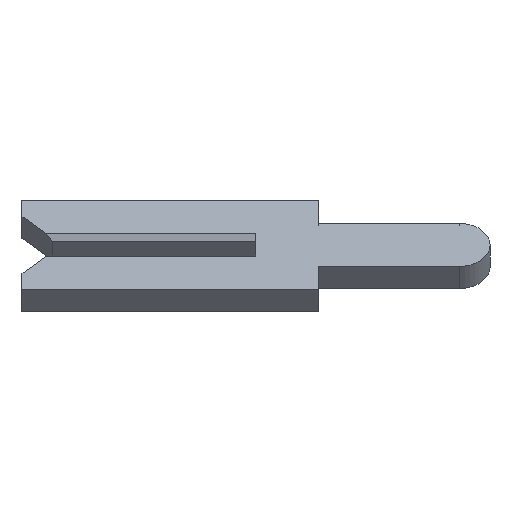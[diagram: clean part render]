
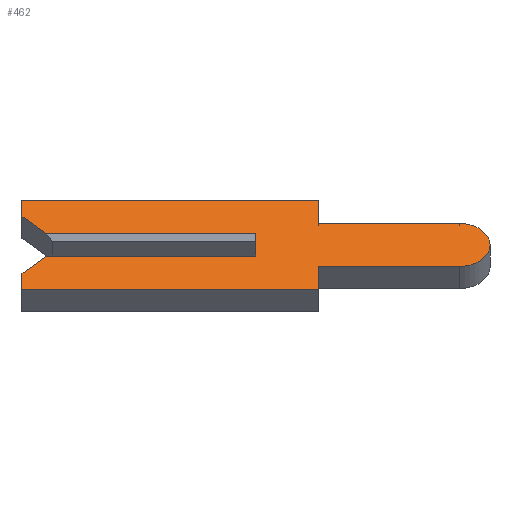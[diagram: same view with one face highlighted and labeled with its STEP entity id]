
A CAD part, left-side view. The second image highlights one B-rep face of the part: STEP entity #462.
In plain terms, the highlighted face is planar.
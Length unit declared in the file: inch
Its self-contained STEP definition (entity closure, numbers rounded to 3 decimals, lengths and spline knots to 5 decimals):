
#1 = VECTOR ( 'NONE', #434, 39.37008 ) ;
#3 = VERTEX_POINT ( 'NONE', #767 ) ;
#26 = ORIENTED_EDGE ( 'NONE', *, *, #602, .F. ) ;
#40 = CIRCLE ( 'NONE', #353, 0.0195 ) ;
#43 = VERTEX_POINT ( 'NONE', #74 ) ;
#44 = ORIENTED_EDGE ( 'NONE', *, *, #184, .F. ) ;
#53 = LINE ( 'NONE', #195, #673 ) ;
#74 = CARTESIAN_POINT ( 'NONE',  ( -0.01, 0.15, 0.04 ) ) ;
#82 = VERTEX_POINT ( 'NONE', #422 ) ;
#83 = CARTESIAN_POINT ( 'NONE',  ( -0.01, 0., 0.0065 ) ) ;
#100 = VECTOR ( 'NONE', #306, 39.37008 ) ;
#101 = ORIENTED_EDGE ( 'NONE', *, *, #229, .F. ) ;
#118 = AXIS2_PLACEMENT_3D ( 'NONE', #884, #601, #881 ) ;
#122 = VECTOR ( 'NONE', #298, 39.37008 ) ;
#135 = VERTEX_POINT ( 'NONE', #213 ) ;
#138 = CARTESIAN_POINT ( 'NONE',  ( -0.01, -0.1305, -0.0195 ) ) ;
#170 = VERTEX_POINT ( 'NONE', #138 ) ;
#176 = VECTOR ( 'NONE', #814, 39.37008 ) ;
#178 = CARTESIAN_POINT ( 'NONE',  ( -0.01, 0., 0.01 ) ) ;
#182 = VERTEX_POINT ( 'NONE', #630 ) ;
#184 = EDGE_CURVE ( 'NONE', #135, #82, #272, .T. ) ;
#185 = LINE ( 'NONE', #519, #402 ) ;
#188 = DIRECTION ( 'NONE',  ( 0., 0., -1. ) ) ;
#191 = ORIENTED_EDGE ( 'NONE', *, *, #483, .F. ) ;
#195 = CARTESIAN_POINT ( 'NONE',  ( -0.01, 0.15, -0.026 ) ) ;
#213 = CARTESIAN_POINT ( 'NONE',  ( -0.01, -0.04, 0.0195 ) ) ;
#216 = ORIENTED_EDGE ( 'NONE', *, *, #458, .F. ) ;
#226 = VERTEX_POINT ( 'NONE', #854 ) ;
#229 = EDGE_CURVE ( 'NONE', #720, #135, #419, .T. ) ;
#232 = CARTESIAN_POINT ( 'NONE',  ( -0.01, -0.1305, -0.01 ) ) ;
#265 = VERTEX_POINT ( 'NONE', #656 ) ;
#270 = EDGE_CURVE ( 'NONE', #592, #521, #919, .T. ) ;
#272 = LINE ( 'NONE', #704, #344 ) ;
#274 = DIRECTION ( 'NONE',  ( 0., -1., 0. ) ) ;
#289 = DIRECTION ( 'NONE',  ( 0., 0.707, 0.707 ) ) ;
#298 = DIRECTION ( 'NONE',  ( 0., -1., 0. ) ) ;
#300 = LINE ( 'NONE', #789, #864 ) ;
#304 = EDGE_CURVE ( 'NONE', #898, #521, #300, .T. ) ;
#306 = DIRECTION ( 'NONE',  ( 0., 0., 1. ) ) ;
#307 = LINE ( 'NONE', #452, #176 ) ;
#321 = PLANE ( 'NONE',  #118 ) ;
#324 = VERTEX_POINT ( 'NONE', #802 ) ;
#336 = EDGE_LOOP ( 'NONE', ( #764, #420, #840, #391, #382, #26, #191, #866, #369, #44, #101, #660, #755, #216 ) ) ;
#338 = DIRECTION ( 'NONE',  ( 0., 0., 1. ) ) ;
#344 = VECTOR ( 'NONE', #274, 39.37008 ) ;
#347 = VECTOR ( 'NONE', #466, 39.37008 ) ;
#352 = CARTESIAN_POINT ( 'NONE',  ( -0.01, -0.04, 0.04 ) ) ;
#353 = AXIS2_PLACEMENT_3D ( 'NONE', #619, #615, #188 ) ;
#360 = LINE ( 'NONE', #461, #439 ) ;
#366 = CARTESIAN_POINT ( 'NONE',  ( -0.01, 0.15, 0.04 ) ) ;
#369 = ORIENTED_EDGE ( 'NONE', *, *, #695, .F. ) ;
#372 = LINE ( 'NONE', #232, #347 ) ;
#381 = EDGE_CURVE ( 'NONE', #226, #43, #467, .T. ) ;
#382 = ORIENTED_EDGE ( 'NONE', *, *, #910, .F. ) ;
#387 = CARTESIAN_POINT ( 'NONE',  ( -0.01, 0., -0.01 ) ) ;
#391 = ORIENTED_EDGE ( 'NONE', *, *, #530, .F. ) ;
#398 = VECTOR ( 'NONE', #869, 39.37008 ) ;
#402 = VECTOR ( 'NONE', #525, 39.37008 ) ;
#403 = CARTESIAN_POINT ( 'NONE',  ( -0.01, 0.134, 0.01 ) ) ;
#408 = VECTOR ( 'NONE', #504, 39.37008 ) ;
#419 = LINE ( 'NONE', #352, #1 ) ;
#420 = ORIENTED_EDGE ( 'NONE', *, *, #270, .F. ) ;
#422 = CARTESIAN_POINT ( 'NONE',  ( -0.01, -0.1305, 0.0195 ) ) ;
#424 = EDGE_CURVE ( 'NONE', #43, #720, #883, .T. ) ;
#430 = CARTESIAN_POINT ( 'NONE',  ( -0.01, -0.04, -0.0195 ) ) ;
#434 = DIRECTION ( 'NONE',  ( 0., 0., -1. ) ) ;
#438 = EDGE_CURVE ( 'NONE', #170, #324, #917, .T. ) ;
#439 = VECTOR ( 'NONE', #671, 39.37008 ) ;
#452 = CARTESIAN_POINT ( 'NONE',  ( -0.01, -0.04, -0.04 ) ) ;
#458 = EDGE_CURVE ( 'NONE', #898, #226, #740, .T. ) ;
#461 = CARTESIAN_POINT ( 'NONE',  ( -0.01, 0.15, -0.04 ) ) ;
#462 = ADVANCED_FACE ( 'NONE', ( #580 ), #321, .F. ) ;
#466 = DIRECTION ( 'NONE',  ( 0., -1., 0. ) ) ;
#467 = LINE ( 'NONE', #731, #100 ) ;
#483 = EDGE_CURVE ( 'NONE', #324, #182, #307, .T. ) ;
#504 = DIRECTION ( 'NONE',  ( 0., 1., 0. ) ) ;
#519 = CARTESIAN_POINT ( 'NONE',  ( -0.01, 0.1305, -0.0065 ) ) ;
#521 = VERTEX_POINT ( 'NONE', #178 ) ;
#525 = DIRECTION ( 'NONE',  ( 0., -0.707, 0.707 ) ) ;
#530 = EDGE_CURVE ( 'NONE', #265, #839, #185, .T. ) ;
#554 = CARTESIAN_POINT ( 'NONE',  ( -0.01, 0.134, -0.01 ) ) ;
#580 = FACE_OUTER_BOUND ( 'NONE', #336, .T. ) ;
#592 = VERTEX_POINT ( 'NONE', #387 ) ;
#601 = DIRECTION ( 'NONE',  ( 1., 0., 0. ) ) ;
#602 = EDGE_CURVE ( 'NONE', #182, #3, #360, .T. ) ;
#615 = DIRECTION ( 'NONE',  ( 1., 0., 0. ) ) ;
#619 = CARTESIAN_POINT ( 'NONE',  ( -0.01, -0.1305, 0. ) ) ;
#630 = CARTESIAN_POINT ( 'NONE',  ( -0.01, -0.04, -0.04 ) ) ;
#650 = EDGE_CURVE ( 'NONE', #839, #592, #372, .T. ) ;
#656 = CARTESIAN_POINT ( 'NONE',  ( -0.01, 0.15, -0.026 ) ) ;
#659 = DIRECTION ( 'NONE',  ( 0., -1., 0. ) ) ;
#660 = ORIENTED_EDGE ( 'NONE', *, *, #424, .F. ) ;
#671 = DIRECTION ( 'NONE',  ( 0., 1., 0. ) ) ;
#673 = VECTOR ( 'NONE', #338, 39.37008 ) ;
#689 = CARTESIAN_POINT ( 'NONE',  ( -0.01, -0.04, 0.04 ) ) ;
#695 = EDGE_CURVE ( 'NONE', #82, #170, #40, .T. ) ;
#704 = CARTESIAN_POINT ( 'NONE',  ( -0.01, -0.04, 0.0195 ) ) ;
#720 = VERTEX_POINT ( 'NONE', #689 ) ;
#731 = CARTESIAN_POINT ( 'NONE',  ( -0.01, 0.15, 0.026 ) ) ;
#740 = LINE ( 'NONE', #797, #902 ) ;
#755 = ORIENTED_EDGE ( 'NONE', *, *, #381, .F. ) ;
#764 = ORIENTED_EDGE ( 'NONE', *, *, #304, .T. ) ;
#767 = CARTESIAN_POINT ( 'NONE',  ( -0.01, 0.15, -0.04 ) ) ;
#789 = CARTESIAN_POINT ( 'NONE',  ( -0.01, 0.15, 0.01 ) ) ;
#797 = CARTESIAN_POINT ( 'NONE',  ( -0.01, 0.1305, 0.0065 ) ) ;
#802 = CARTESIAN_POINT ( 'NONE',  ( -0.01, -0.04, -0.0195 ) ) ;
#814 = DIRECTION ( 'NONE',  ( 0., 0., -1. ) ) ;
#839 = VERTEX_POINT ( 'NONE', #554 ) ;
#840 = ORIENTED_EDGE ( 'NONE', *, *, #650, .F. ) ;
#854 = CARTESIAN_POINT ( 'NONE',  ( -0.01, 0.15, 0.026 ) ) ;
#864 = VECTOR ( 'NONE', #659, 39.37008 ) ;
#866 = ORIENTED_EDGE ( 'NONE', *, *, #438, .F. ) ;
#869 = DIRECTION ( 'NONE',  ( 0., 0., 1. ) ) ;
#881 = DIRECTION ( 'NONE',  ( 0., 0., -1. ) ) ;
#883 = LINE ( 'NONE', #366, #122 ) ;
#884 = CARTESIAN_POINT ( 'NONE',  ( -0.01, -0.1305, 0. ) ) ;
#898 = VERTEX_POINT ( 'NONE', #403 ) ;
#902 = VECTOR ( 'NONE', #289, 39.37008 ) ;
#910 = EDGE_CURVE ( 'NONE', #3, #265, #53, .T. ) ;
#917 = LINE ( 'NONE', #430, #408 ) ;
#919 = LINE ( 'NONE', #83, #398 ) ;
